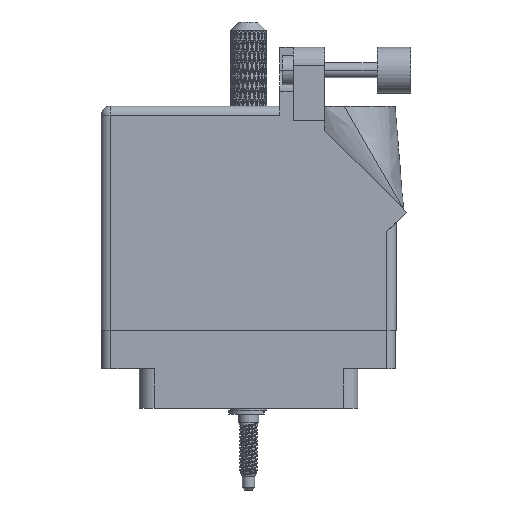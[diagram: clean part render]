
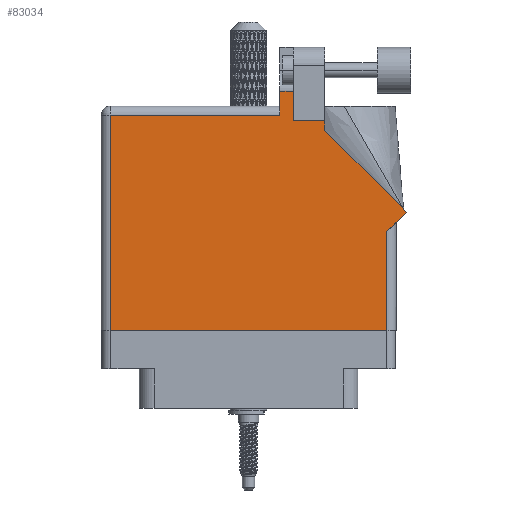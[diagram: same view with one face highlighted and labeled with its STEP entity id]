
A CAD part, front view. The second image highlights one B-rep face of the part: STEP entity #83034.
In plain terms, the highlighted face is planar.
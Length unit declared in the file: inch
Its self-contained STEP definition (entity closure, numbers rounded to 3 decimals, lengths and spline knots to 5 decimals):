
#1074 = DIRECTION ( 'NONE',  ( 0.707, 0.707, 0. ) ) ;
#1141 = CARTESIAN_POINT ( 'NONE',  ( 0.062, 0., 0. ) ) ;
#1496 = DIRECTION ( 'NONE',  ( 0., -1., 0. ) ) ;
#2410 = VECTOR ( 'NONE', #36478, 39.37008 ) ;
#3333 = VECTOR ( 'NONE', #95210, 39.37008 ) ;
#4410 = CARTESIAN_POINT ( 'NONE',  ( 1.217, 1.468, 0. ) ) ;
#8255 = EDGE_CURVE ( 'NONE', #35100, #48908, #35496, .T. ) ;
#9088 = VERTEX_POINT ( 'NONE', #36827 ) ;
#12349 = DIRECTION ( 'NONE',  ( -1., 0., 0. ) ) ;
#12601 = LINE ( 'NONE', #28553, #89998 ) ;
#14276 = CARTESIAN_POINT ( 'NONE',  ( 1.311, 1.6315, 0. ) ) ;
#14495 = ORIENTED_EDGE ( 'NONE', *, *, #90787, .T. ) ;
#17244 = LINE ( 'NONE', #50563, #70495 ) ;
#20304 = CARTESIAN_POINT ( 'NONE',  ( 1.64177, 1.6315, 0. ) ) ;
#20907 = ORIENTED_EDGE ( 'NONE', *, *, #81272, .T. ) ;
#21149 = VECTOR ( 'NONE', #64917, 39.37008 ) ;
#22370 = ORIENTED_EDGE ( 'NONE', *, *, #75552, .T. ) ;
#23157 = CARTESIAN_POINT ( 'NONE',  ( 0., 0., 0. ) ) ;
#23176 = EDGE_CURVE ( 'NONE', #52476, #36422, #58997, .T. ) ;
#25897 = LINE ( 'NONE', #94871, #44884 ) ;
#26670 = CARTESIAN_POINT ( 'NONE',  ( 1.948, 0., 0. ) ) ;
#27428 = DIRECTION ( 'NONE',  ( 0., 1., 0. ) ) ;
#27978 = VECTOR ( 'NONE', #1074, 39.37008 ) ;
#28553 = CARTESIAN_POINT ( 'NONE',  ( 1.948, 0.737, 0. ) ) ;
#30157 = VERTEX_POINT ( 'NONE', #14276 ) ;
#30533 = AXIS2_PLACEMENT_3D ( 'NONE', #52326, #69068, #12349 ) ;
#30640 = VERTEX_POINT ( 'NONE', #97741 ) ;
#31181 = LINE ( 'NONE', #62548, #3333 ) ;
#31560 = LINE ( 'NONE', #20304, #2410 ) ;
#32283 = CARTESIAN_POINT ( 'NONE',  ( 1.524, 1.36442, 0. ) ) ;
#34303 = VERTEX_POINT ( 'NONE', #26670 ) ;
#35100 = VERTEX_POINT ( 'NONE', #36290 ) ;
#35496 = LINE ( 'NONE', #98158, #27978 ) ;
#36290 = CARTESIAN_POINT ( 'NONE',  ( 1.948, 0.675, 0. ) ) ;
#36422 = VERTEX_POINT ( 'NONE', #37482 ) ;
#36478 = DIRECTION ( 'NONE',  ( -1., 0., 0. ) ) ;
#36604 = DIRECTION ( 'NONE',  ( 0., 1., 0. ) ) ;
#36827 = CARTESIAN_POINT ( 'NONE',  ( 0.062, 0., 0. ) ) ;
#37482 = CARTESIAN_POINT ( 'NONE',  ( 0.062, 1.468, 0. ) ) ;
#37877 = EDGE_CURVE ( 'NONE', #34303, #35100, #12601, .T. ) ;
#44884 = VECTOR ( 'NONE', #88111, 39.37008 ) ;
#47452 = ORIENTED_EDGE ( 'NONE', *, *, #23176, .T. ) ;
#48908 = VERTEX_POINT ( 'NONE', #62885 ) ;
#49805 = VECTOR ( 'NONE', #104704, 39.37008 ) ;
#50563 = CARTESIAN_POINT ( 'NONE',  ( 1.311, 1.43, 0. ) ) ;
#52326 = CARTESIAN_POINT ( 'NONE',  ( 0., 1.53, 0. ) ) ;
#52400 = FACE_OUTER_BOUND ( 'NONE', #53273, .T. ) ;
#52476 = VERTEX_POINT ( 'NONE', #4410 ) ;
#53194 = VERTEX_POINT ( 'NONE', #92808 ) ;
#53273 = EDGE_LOOP ( 'NONE', ( #104141, #65954, #69739, #47452, #20907, #101043, #56665, #56699, #66534, #22370, #14495 ) ) ;
#54404 = LINE ( 'NONE', #66790, #89938 ) ;
#55910 = DIRECTION ( 'NONE',  ( -1., 0., 0. ) ) ;
#55960 = EDGE_CURVE ( 'NONE', #48908, #86308, #31181, .T. ) ;
#56665 = ORIENTED_EDGE ( 'NONE', *, *, #37877, .T. ) ;
#56699 = ORIENTED_EDGE ( 'NONE', *, *, #8255, .T. ) ;
#58997 = LINE ( 'NONE', #97044, #74325 ) ;
#60050 = LINE ( 'NONE', #23157, #49805 ) ;
#62548 = CARTESIAN_POINT ( 'NONE',  ( 2.08071, 0.80771, 0. ) ) ;
#62721 = CARTESIAN_POINT ( 'NONE',  ( 1.311, 1.43, 0. ) ) ;
#62885 = CARTESIAN_POINT ( 'NONE',  ( 2.08071, 0.80771, 0. ) ) ;
#64917 = DIRECTION ( 'NONE',  ( 0., -1., 0. ) ) ;
#65954 = ORIENTED_EDGE ( 'NONE', *, *, #70254, .T. ) ;
#66534 = ORIENTED_EDGE ( 'NONE', *, *, #55960, .T. ) ;
#66790 = CARTESIAN_POINT ( 'NONE',  ( 1.524, 1.36442, 0. ) ) ;
#68107 = LINE ( 'NONE', #73120, #21149 ) ;
#69068 = DIRECTION ( 'NONE',  ( 0., 0., -1. ) ) ;
#69421 = PLANE ( 'NONE',  #30533 ) ;
#69739 = ORIENTED_EDGE ( 'NONE', *, *, #97144, .T. ) ;
#70254 = EDGE_CURVE ( 'NONE', #30157, #30640, #31560, .T. ) ;
#70495 = VECTOR ( 'NONE', #93204, 39.37008 ) ;
#73120 = CARTESIAN_POINT ( 'NONE',  ( 1.217, 1.53, 0. ) ) ;
#74325 = VECTOR ( 'NONE', #55910, 39.37008 ) ;
#75552 = EDGE_CURVE ( 'NONE', #86308, #53194, #54404, .T. ) ;
#77272 = VERTEX_POINT ( 'NONE', #62721 ) ;
#80123 = LINE ( 'NONE', #1141, #82659 ) ;
#81272 = EDGE_CURVE ( 'NONE', #36422, #9088, #80123, .T. ) ;
#82659 = VECTOR ( 'NONE', #1496, 39.37008 ) ;
#83034 = ADVANCED_FACE ( 'NONE', ( #52400 ), #69421, .F. ) ;
#86308 = VERTEX_POINT ( 'NONE', #32283 ) ;
#88111 = DIRECTION ( 'NONE',  ( -1., 0., 0. ) ) ;
#89938 = VECTOR ( 'NONE', #27428, 39.37008 ) ;
#89998 = VECTOR ( 'NONE', #36604, 39.37008 ) ;
#90787 = EDGE_CURVE ( 'NONE', #53194, #77272, #25897, .T. ) ;
#91276 = EDGE_CURVE ( 'NONE', #9088, #34303, #60050, .T. ) ;
#92808 = CARTESIAN_POINT ( 'NONE',  ( 1.524, 1.43, 0. ) ) ;
#93005 = EDGE_CURVE ( 'NONE', #77272, #30157, #17244, .T. ) ;
#93204 = DIRECTION ( 'NONE',  ( 0., 1., 0. ) ) ;
#94871 = CARTESIAN_POINT ( 'NONE',  ( 1.524, 1.43, 0. ) ) ;
#95210 = DIRECTION ( 'NONE',  ( -0.707, 0.707, 0. ) ) ;
#97044 = CARTESIAN_POINT ( 'NONE',  ( 0., 1.468, 0. ) ) ;
#97144 = EDGE_CURVE ( 'NONE', #30640, #52476, #68107, .T. ) ;
#97741 = CARTESIAN_POINT ( 'NONE',  ( 1.217, 1.6315, 0. ) ) ;
#98158 = CARTESIAN_POINT ( 'NONE',  ( 2.01, 0.737, 0. ) ) ;
#101043 = ORIENTED_EDGE ( 'NONE', *, *, #91276, .T. ) ;
#104141 = ORIENTED_EDGE ( 'NONE', *, *, #93005, .T. ) ;
#104704 = DIRECTION ( 'NONE',  ( 1., 0., 0. ) ) ;
